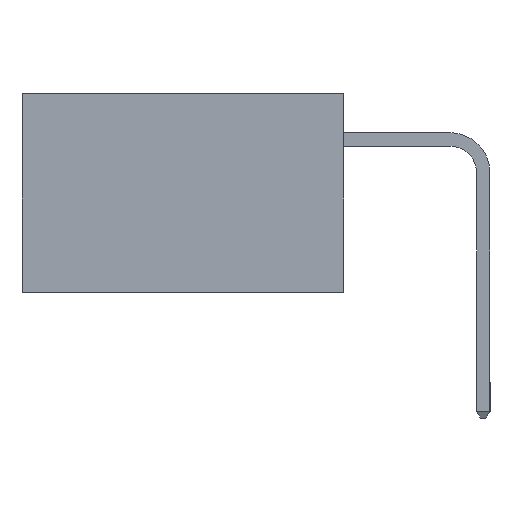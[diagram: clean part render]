
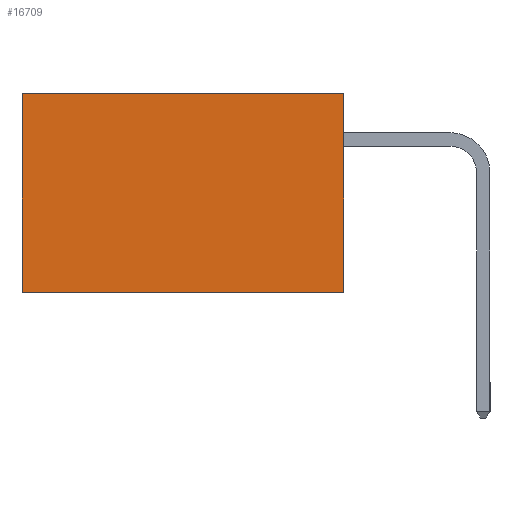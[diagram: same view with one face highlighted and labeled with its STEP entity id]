
A CAD part, left-side view. The second image highlights one B-rep face of the part: STEP entity #16709.
In plain terms, the highlighted planar face has unit normal (-1, 0, 0).
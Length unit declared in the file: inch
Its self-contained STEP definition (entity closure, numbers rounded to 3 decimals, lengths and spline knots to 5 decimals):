
#376 = CARTESIAN_POINT ( 'NONE',  ( 0.298, 0., -0.37 ) ) ;
#1449 = DIRECTION ( 'NONE',  ( 0., 0., -1. ) ) ;
#2756 = VECTOR ( 'NONE', #25665, 39.37008 ) ;
#3954 = ORIENTED_EDGE ( 'NONE', *, *, #15929, .F. ) ;
#4430 = CARTESIAN_POINT ( 'NONE',  ( 0.298, 0.6, 0. ) ) ;
#5330 = CARTESIAN_POINT ( 'NONE',  ( 0.298, 0., 0. ) ) ;
#6149 = CARTESIAN_POINT ( 'NONE',  ( 0.298, 0., 0. ) ) ;
#6783 = CARTESIAN_POINT ( 'NONE',  ( 0.298, 0.6, -0.37 ) ) ;
#6866 = LINE ( 'NONE', #4430, #18721 ) ;
#6876 = ORIENTED_EDGE ( 'NONE', *, *, #25873, .T. ) ;
#6918 = VERTEX_POINT ( 'NONE', #6783 ) ;
#7778 = VERTEX_POINT ( 'NONE', #12378 ) ;
#8615 = AXIS2_PLACEMENT_3D ( 'NONE', #6149, #25125, #1449 ) ;
#9557 = LINE ( 'NONE', #14589, #20365 ) ;
#9813 = DIRECTION ( 'NONE',  ( 0., 0., -1. ) ) ;
#11004 = DIRECTION ( 'NONE',  ( 0., 0., -1. ) ) ;
#11791 = VERTEX_POINT ( 'NONE', #19434 ) ;
#11897 = VERTEX_POINT ( 'NONE', #376 ) ;
#12378 = CARTESIAN_POINT ( 'NONE',  ( 0.298, 0.6, 0. ) ) ;
#12637 = PLANE ( 'NONE',  #8615 ) ;
#12691 = LINE ( 'NONE', #5330, #23108 ) ;
#13070 = CARTESIAN_POINT ( 'NONE',  ( 0.298, 0., 0. ) ) ;
#13788 = ORIENTED_EDGE ( 'NONE', *, *, #13912, .F. ) ;
#13912 = EDGE_CURVE ( 'NONE', #11897, #6918, #9557, .T. ) ;
#14339 = FACE_OUTER_BOUND ( 'NONE', #16893, .T. ) ;
#14589 = CARTESIAN_POINT ( 'NONE',  ( 0.298, 0., -0.37 ) ) ;
#15929 = EDGE_CURVE ( 'NONE', #11791, #11897, #12691, .T. ) ;
#16650 = LINE ( 'NONE', #13070, #2756 ) ;
#16709 = ADVANCED_FACE ( 'NONE', ( #14339 ), #12637, .F. ) ;
#16755 = DIRECTION ( 'NONE',  ( 0., 1., 0. ) ) ;
#16893 = EDGE_LOOP ( 'NONE', ( #6876, #13788, #3954, #19295 ) ) ;
#18721 = VECTOR ( 'NONE', #11004, 39.37008 ) ;
#19295 = ORIENTED_EDGE ( 'NONE', *, *, #26452, .T. ) ;
#19434 = CARTESIAN_POINT ( 'NONE',  ( 0.298, 0., 0. ) ) ;
#20365 = VECTOR ( 'NONE', #16755, 39.37008 ) ;
#23108 = VECTOR ( 'NONE', #9813, 39.37008 ) ;
#25125 = DIRECTION ( 'NONE',  ( 1., 0., 0. ) ) ;
#25665 = DIRECTION ( 'NONE',  ( 0., 1., 0. ) ) ;
#25873 = EDGE_CURVE ( 'NONE', #7778, #6918, #6866, .T. ) ;
#26452 = EDGE_CURVE ( 'NONE', #11791, #7778, #16650, .T. ) ;
